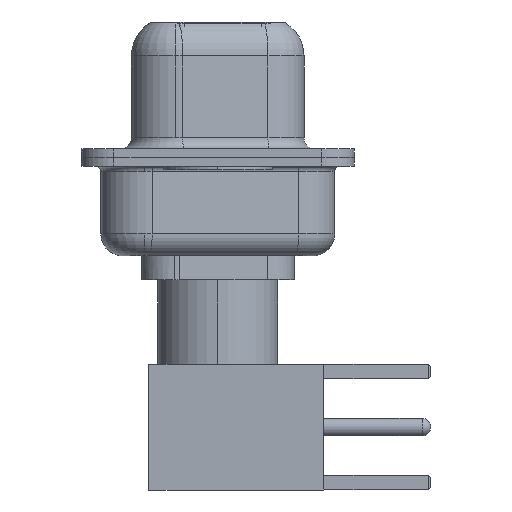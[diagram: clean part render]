
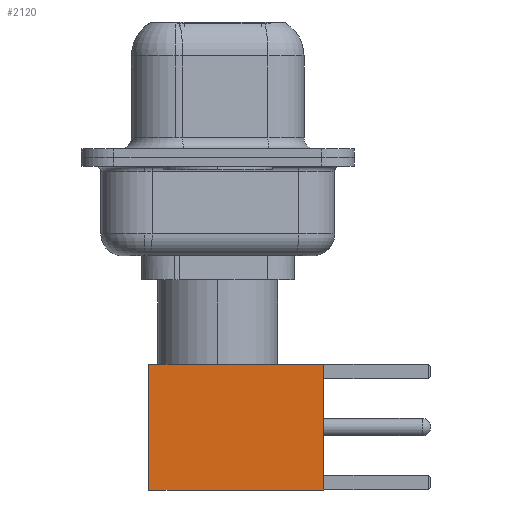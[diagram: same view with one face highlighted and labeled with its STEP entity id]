
A CAD part, left-side view. The second image highlights one B-rep face of the part: STEP entity #2120.
In plain terms, the highlighted face is planar.
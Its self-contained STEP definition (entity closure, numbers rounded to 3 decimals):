
#191 = DIRECTION ( 'NONE',  ( 0., 0., -1. ) ) ;
#226 = DIRECTION ( 'NONE',  ( -1., 0., 0. ) ) ;
#676 = DIRECTION ( 'NONE',  ( 0., 1., 0. ) ) ;
#871 = ORIENTED_EDGE ( 'NONE', *, *, #7327, .F. ) ;
#1084 = AXIS2_PLACEMENT_3D ( 'NONE', #12501, #676, #7757 ) ;
#1119 = VECTOR ( 'NONE', #5675, 1000. ) ;
#1828 = ORIENTED_EDGE ( 'NONE', *, *, #9569, .F. ) ;
#2011 = EDGE_LOOP ( 'NONE', ( #9655, #14385, #1828, #871 ) ) ;
#2120 = ADVANCED_FACE ( 'NONE', ( #7833 ), #10293, .T. ) ;
#2485 = DIRECTION ( 'NONE',  ( -1., 0., 0. ) ) ;
#3787 = EDGE_CURVE ( 'NONE', #11778, #7784, #9246, .T. ) ;
#5675 = DIRECTION ( 'NONE',  ( 0., 0., -1. ) ) ;
#6866 = CARTESIAN_POINT ( 'NONE',  ( 2.875, 2.875, 8. ) ) ;
#6976 = VERTEX_POINT ( 'NONE', #7689 ) ;
#7118 = CARTESIAN_POINT ( 'NONE',  ( 0., 2.875, 0. ) ) ;
#7304 = VECTOR ( 'NONE', #226, 1000. ) ;
#7327 = EDGE_CURVE ( 'NONE', #11778, #8088, #9691, .T. ) ;
#7689 = CARTESIAN_POINT ( 'NONE',  ( -2.875, 2.875, 0. ) ) ;
#7757 = DIRECTION ( 'NONE',  ( 0., 0., 1. ) ) ;
#7784 = VERTEX_POINT ( 'NONE', #9543 ) ;
#7833 = FACE_OUTER_BOUND ( 'NONE', #2011, .T. ) ;
#8048 = CARTESIAN_POINT ( 'NONE',  ( -2.875, 2.875, 8. ) ) ;
#8088 = VERTEX_POINT ( 'NONE', #8048 ) ;
#8195 = EDGE_CURVE ( 'NONE', #7784, #6976, #11715, .T. ) ;
#8247 = CARTESIAN_POINT ( 'NONE',  ( 2.875, 2.875, 0. ) ) ;
#8553 = CARTESIAN_POINT ( 'NONE',  ( 0., 2.875, 8. ) ) ;
#9246 = LINE ( 'NONE', #8247, #1119 ) ;
#9429 = LINE ( 'NONE', #11719, #13858 ) ;
#9543 = CARTESIAN_POINT ( 'NONE',  ( 2.875, 2.875, 0. ) ) ;
#9569 = EDGE_CURVE ( 'NONE', #8088, #6976, #9429, .T. ) ;
#9655 = ORIENTED_EDGE ( 'NONE', *, *, #3787, .T. ) ;
#9687 = VECTOR ( 'NONE', #2485, 1000. ) ;
#9691 = LINE ( 'NONE', #8553, #7304 ) ;
#10293 = PLANE ( 'NONE',  #1084 ) ;
#11715 = LINE ( 'NONE', #7118, #9687 ) ;
#11719 = CARTESIAN_POINT ( 'NONE',  ( -2.875, 2.875, 0. ) ) ;
#11778 = VERTEX_POINT ( 'NONE', #6866 ) ;
#12501 = CARTESIAN_POINT ( 'NONE',  ( 2.875, 2.875, 0. ) ) ;
#13858 = VECTOR ( 'NONE', #191, 1000. ) ;
#14385 = ORIENTED_EDGE ( 'NONE', *, *, #8195, .T. ) ;
